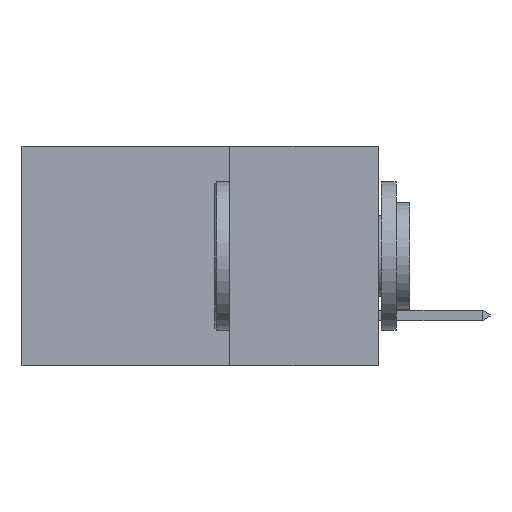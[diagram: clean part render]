
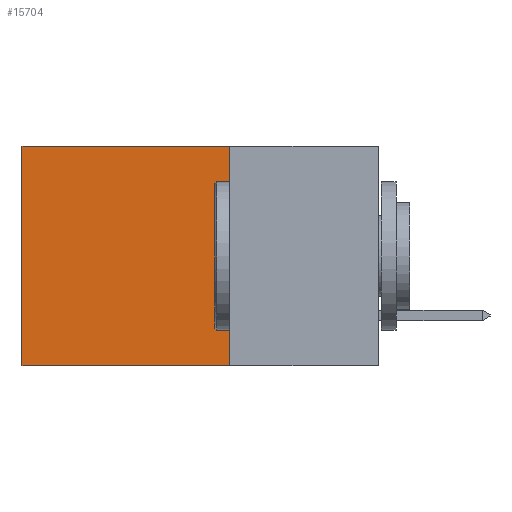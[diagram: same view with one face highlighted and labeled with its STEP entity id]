
A CAD part, left-side view. The second image highlights one B-rep face of the part: STEP entity #15704.
In plain terms, the highlighted planar face has unit normal (-1, 0, 0).
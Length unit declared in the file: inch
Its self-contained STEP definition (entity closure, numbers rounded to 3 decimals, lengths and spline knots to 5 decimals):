
#517 = CARTESIAN_POINT ( 'NONE',  ( 0.2615, 0.25, -0.37 ) ) ;
#584 = CARTESIAN_POINT ( 'NONE',  ( 0.2615, 0.25, -0.37 ) ) ;
#1256 = CARTESIAN_POINT ( 'NONE',  ( 0.2615, 0.6, -0.37 ) ) ;
#1468 = VECTOR ( 'NONE', #1885, 39.37008 ) ;
#1852 = EDGE_LOOP ( 'NONE', ( #8949, #2208, #7621, #10333 ) ) ;
#1885 = DIRECTION ( 'NONE',  ( 0., 0., -1. ) ) ;
#1944 = DIRECTION ( 'NONE',  ( 1., 0., 0. ) ) ;
#2208 = ORIENTED_EDGE ( 'NONE', *, *, #14449, .F. ) ;
#3961 = VERTEX_POINT ( 'NONE', #6666 ) ;
#4167 = VECTOR ( 'NONE', #5948, 39.37008 ) ;
#5787 = VERTEX_POINT ( 'NONE', #1256 ) ;
#5948 = DIRECTION ( 'NONE',  ( 0., 0., -1. ) ) ;
#6666 = CARTESIAN_POINT ( 'NONE',  ( 0.2615, 0.25, -0.37 ) ) ;
#7202 = CARTESIAN_POINT ( 'NONE',  ( 0.2615, 0.25, -0.37 ) ) ;
#7517 = LINE ( 'NONE', #7202, #14441 ) ;
#7621 = ORIENTED_EDGE ( 'NONE', *, *, #15678, .F. ) ;
#7869 = LINE ( 'NONE', #16940, #4167 ) ;
#8300 = FACE_OUTER_BOUND ( 'NONE', #1852, .T. ) ;
#8949 = ORIENTED_EDGE ( 'NONE', *, *, #11907, .T. ) ;
#9092 = VERTEX_POINT ( 'NONE', #12432 ) ;
#9425 = VERTEX_POINT ( 'NONE', #9652 ) ;
#9652 = CARTESIAN_POINT ( 'NONE',  ( 0.2615, 0.25, 0. ) ) ;
#10174 = PLANE ( 'NONE',  #16035 ) ;
#10299 = CARTESIAN_POINT ( 'NONE',  ( 0.2615, 0.25, 0. ) ) ;
#10333 = ORIENTED_EDGE ( 'NONE', *, *, #13203, .T. ) ;
#11256 = LINE ( 'NONE', #10299, #14894 ) ;
#11585 = DIRECTION ( 'NONE',  ( 0., 0., -1. ) ) ;
#11907 = EDGE_CURVE ( 'NONE', #9092, #5787, #7869, .T. ) ;
#12432 = CARTESIAN_POINT ( 'NONE',  ( 0.2615, 0.6, 0. ) ) ;
#12469 = LINE ( 'NONE', #517, #1468 ) ;
#13114 = DIRECTION ( 'NONE',  ( 0., 1., 0. ) ) ;
#13203 = EDGE_CURVE ( 'NONE', #9425, #9092, #11256, .T. ) ;
#14441 = VECTOR ( 'NONE', #16758, 39.37008 ) ;
#14449 = EDGE_CURVE ( 'NONE', #3961, #5787, #7517, .T. ) ;
#14894 = VECTOR ( 'NONE', #13114, 39.37008 ) ;
#15678 = EDGE_CURVE ( 'NONE', #9425, #3961, #12469, .T. ) ;
#15704 = ADVANCED_FACE ( 'NONE', ( #8300 ), #10174, .F. ) ;
#16035 = AXIS2_PLACEMENT_3D ( 'NONE', #584, #1944, #11585 ) ;
#16758 = DIRECTION ( 'NONE',  ( 0., 1., 0. ) ) ;
#16940 = CARTESIAN_POINT ( 'NONE',  ( 0.2615, 0.6, -0.37 ) ) ;
